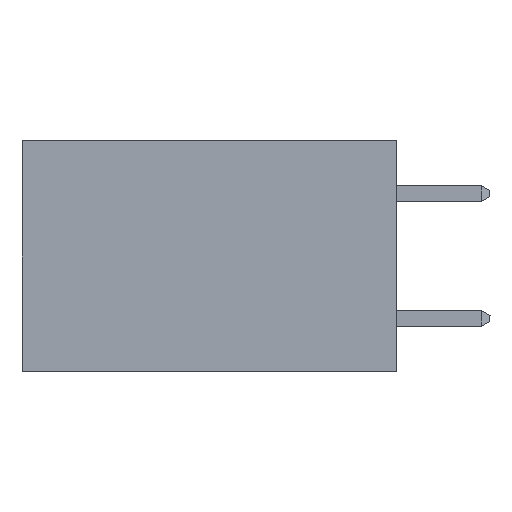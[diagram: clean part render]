
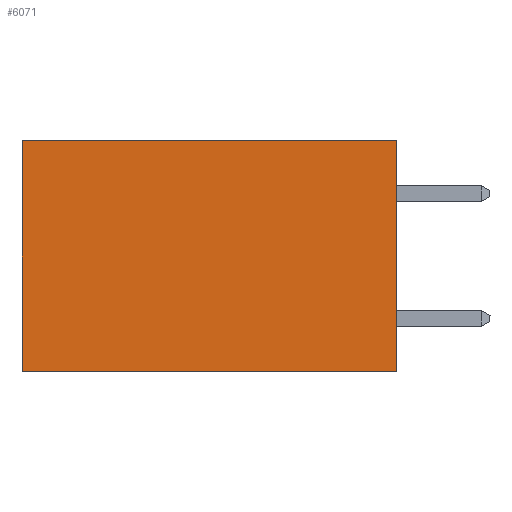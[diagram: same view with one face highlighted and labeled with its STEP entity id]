
A CAD part, left-side view. The second image highlights one B-rep face of the part: STEP entity #6071.
In plain terms, the highlighted planar face has unit normal (-1, 0, 0).
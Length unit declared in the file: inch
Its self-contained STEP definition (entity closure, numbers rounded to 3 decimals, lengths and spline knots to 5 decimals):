
#589 = EDGE_CURVE ( 'NONE', #17805, #5187, #5889, .T. ) ;
#2460 = DIRECTION ( 'NONE',  ( 0., 0., -1. ) ) ;
#2965 = VERTEX_POINT ( 'NONE', #5513 ) ;
#3172 = VECTOR ( 'NONE', #2460, 39.37008 ) ;
#3789 = EDGE_CURVE ( 'NONE', #2965, #12036, #6638, .T. ) ;
#4605 = VECTOR ( 'NONE', #11132, 39.37008 ) ;
#5187 = VERTEX_POINT ( 'NONE', #8943 ) ;
#5513 = CARTESIAN_POINT ( 'NONE',  ( 0.2615, 0., 0. ) ) ;
#5889 = LINE ( 'NONE', #14574, #9642 ) ;
#6071 = ADVANCED_FACE ( 'NONE', ( #13263 ), #16574, .F. ) ;
#6638 = LINE ( 'NONE', #13994, #13576 ) ;
#6686 = ORIENTED_EDGE ( 'NONE', *, *, #12793, .T. ) ;
#8205 = CARTESIAN_POINT ( 'NONE',  ( 0.2615, 0.6, -0.37 ) ) ;
#8367 = CARTESIAN_POINT ( 'NONE',  ( 0.2615, 0., -0.37 ) ) ;
#8943 = CARTESIAN_POINT ( 'NONE',  ( 0.2615, 0.6, -0.37 ) ) ;
#9642 = VECTOR ( 'NONE', #9786, 39.37008 ) ;
#9668 = CARTESIAN_POINT ( 'NONE',  ( 0.2615, 0.6, 0. ) ) ;
#9786 = DIRECTION ( 'NONE',  ( 0., 1., 0. ) ) ;
#9876 = EDGE_CURVE ( 'NONE', #2965, #17805, #12030, .T. ) ;
#11088 = LINE ( 'NONE', #8205, #3172 ) ;
#11132 = DIRECTION ( 'NONE',  ( 0., 0., -1. ) ) ;
#12030 = LINE ( 'NONE', #8367, #4605 ) ;
#12036 = VERTEX_POINT ( 'NONE', #9668 ) ;
#12318 = EDGE_LOOP ( 'NONE', ( #6686, #14297, #15189, #14271 ) ) ;
#12793 = EDGE_CURVE ( 'NONE', #12036, #5187, #11088, .T. ) ;
#13191 = DIRECTION ( 'NONE',  ( 0., 1., 0. ) ) ;
#13263 = FACE_OUTER_BOUND ( 'NONE', #12318, .T. ) ;
#13576 = VECTOR ( 'NONE', #13191, 39.37008 ) ;
#13994 = CARTESIAN_POINT ( 'NONE',  ( 0.2615, 0., 0. ) ) ;
#14271 = ORIENTED_EDGE ( 'NONE', *, *, #3789, .T. ) ;
#14297 = ORIENTED_EDGE ( 'NONE', *, *, #589, .F. ) ;
#14377 = CARTESIAN_POINT ( 'NONE',  ( 0.2615, 0., -0.37 ) ) ;
#14574 = CARTESIAN_POINT ( 'NONE',  ( 0.2615, 0., -0.37 ) ) ;
#15189 = ORIENTED_EDGE ( 'NONE', *, *, #9876, .F. ) ;
#16026 = AXIS2_PLACEMENT_3D ( 'NONE', #16480, #16375, #16414 ) ;
#16375 = DIRECTION ( 'NONE',  ( 1., 0., 0. ) ) ;
#16414 = DIRECTION ( 'NONE',  ( 0., 0., -1. ) ) ;
#16480 = CARTESIAN_POINT ( 'NONE',  ( 0.2615, 0., -0.37 ) ) ;
#16574 = PLANE ( 'NONE',  #16026 ) ;
#17805 = VERTEX_POINT ( 'NONE', #14377 ) ;
